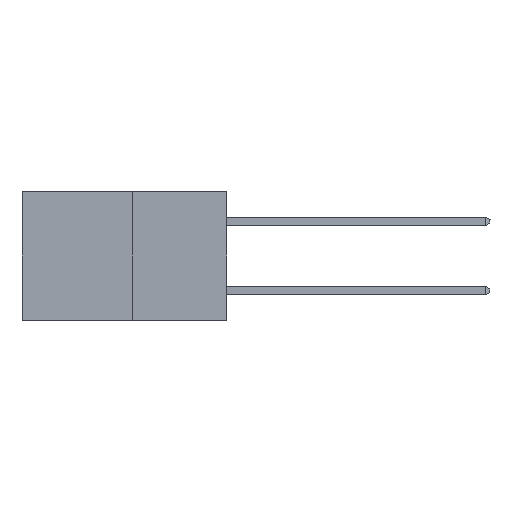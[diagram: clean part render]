
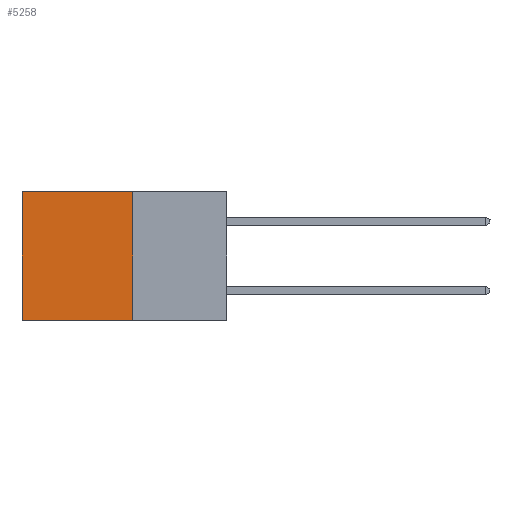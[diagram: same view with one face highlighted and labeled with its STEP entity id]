
A CAD part, left-side view. The second image highlights one B-rep face of the part: STEP entity #5258.
In plain terms, the highlighted planar face has unit normal (-1, 0, 0).
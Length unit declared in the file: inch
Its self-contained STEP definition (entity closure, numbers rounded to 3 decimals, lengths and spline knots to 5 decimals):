
#289 = LINE ( 'NONE', #4469, #4236 ) ;
#646 = VECTOR ( 'NONE', #5575, 39.37008 ) ;
#710 = EDGE_LOOP ( 'NONE', ( #2287, #2326, #2363, #2373 ) ) ;
#1143 = CARTESIAN_POINT ( 'NONE',  ( 0.277, 0.27, 0. ) ) ;
#1310 = CARTESIAN_POINT ( 'NONE',  ( 0.277, 0.27, -0.37 ) ) ;
#1342 = VECTOR ( 'NONE', #3198, 39.37008 ) ;
#1354 = PLANE ( 'NONE',  #7977 ) ;
#1818 = LINE ( 'NONE', #6946, #1342 ) ;
#1849 = EDGE_CURVE ( 'NONE', #4728, #7206, #1818, .T. ) ;
#2287 = ORIENTED_EDGE ( 'NONE', *, *, #4319, .T. ) ;
#2326 = ORIENTED_EDGE ( 'NONE', *, *, #1849, .F. ) ;
#2363 = ORIENTED_EDGE ( 'NONE', *, *, #4249, .F. ) ;
#2373 = ORIENTED_EDGE ( 'NONE', *, *, #4161, .T. ) ;
#2946 = DIRECTION ( 'NONE',  ( 0., 0., -1. ) ) ;
#3198 = DIRECTION ( 'NONE',  ( 0., 1., 0. ) ) ;
#3624 = CARTESIAN_POINT ( 'NONE',  ( 0.277, 0.59, -0.37 ) ) ;
#4161 = EDGE_CURVE ( 'NONE', #4805, #7268, #7668, .T. ) ;
#4236 = VECTOR ( 'NONE', #4441, 39.37008 ) ;
#4249 = EDGE_CURVE ( 'NONE', #4805, #4728, #5439, .T. ) ;
#4319 = EDGE_CURVE ( 'NONE', #7268, #7206, #289, .T. ) ;
#4394 = CARTESIAN_POINT ( 'NONE',  ( 0.277, 0.59, 0. ) ) ;
#4441 = DIRECTION ( 'NONE',  ( 0., 0., -1. ) ) ;
#4469 = CARTESIAN_POINT ( 'NONE',  ( 0.277, 0.59, -0.37 ) ) ;
#4728 = VERTEX_POINT ( 'NONE', #1310 ) ;
#4805 = VERTEX_POINT ( 'NONE', #1143 ) ;
#5121 = DIRECTION ( 'NONE',  ( 0., 0., -1. ) ) ;
#5127 = CARTESIAN_POINT ( 'NONE',  ( 0.277, 0.27, -0.37 ) ) ;
#5258 = ADVANCED_FACE ( 'NONE', ( #5595 ), #1354, .F. ) ;
#5439 = LINE ( 'NONE', #5127, #6708 ) ;
#5575 = DIRECTION ( 'NONE',  ( 0., 1., 0. ) ) ;
#5595 = FACE_OUTER_BOUND ( 'NONE', #710, .T. ) ;
#5641 = CARTESIAN_POINT ( 'NONE',  ( 0.277, 0.27, 0. ) ) ;
#5732 = CARTESIAN_POINT ( 'NONE',  ( 0.277, 0.27, -0.37 ) ) ;
#6708 = VECTOR ( 'NONE', #5121, 39.37008 ) ;
#6795 = DIRECTION ( 'NONE',  ( 1., 0., 0. ) ) ;
#6946 = CARTESIAN_POINT ( 'NONE',  ( 0.277, 0.27, -0.37 ) ) ;
#7206 = VERTEX_POINT ( 'NONE', #3624 ) ;
#7268 = VERTEX_POINT ( 'NONE', #4394 ) ;
#7668 = LINE ( 'NONE', #5641, #646 ) ;
#7977 = AXIS2_PLACEMENT_3D ( 'NONE', #5732, #6795, #2946 ) ;
